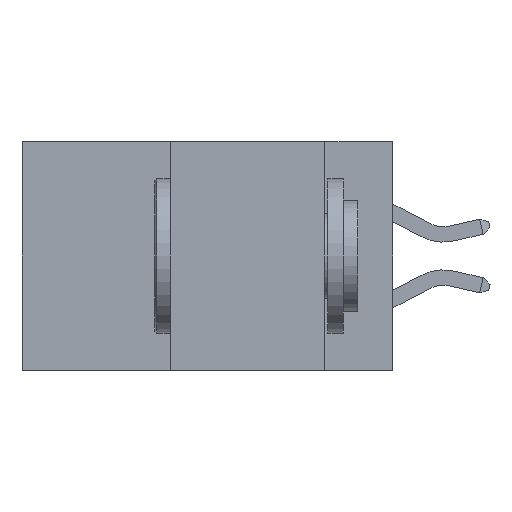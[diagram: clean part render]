
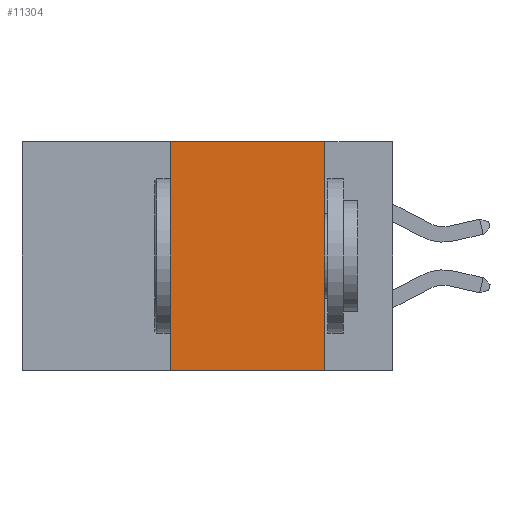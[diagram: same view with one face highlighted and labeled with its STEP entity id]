
A CAD part, left-side view. The second image highlights one B-rep face of the part: STEP entity #11304.
In plain terms, the highlighted planar face has unit normal (-1, 0, 0).
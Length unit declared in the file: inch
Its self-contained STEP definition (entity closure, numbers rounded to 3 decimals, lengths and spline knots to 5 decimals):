
#2167 = VECTOR ( 'NONE', #12149, 39.37008 ) ;
#3644 = EDGE_LOOP ( 'NONE', ( #26997, #8917, #14681, #18625 ) ) ;
#3926 = CARTESIAN_POINT ( 'NONE',  ( 0., 0.11, -0.37 ) ) ;
#5124 = EDGE_CURVE ( 'NONE', #15051, #18869, #25677, .T. ) ;
#5233 = CARTESIAN_POINT ( 'NONE',  ( 0., 0.6, 0. ) ) ;
#6805 = CARTESIAN_POINT ( 'NONE',  ( 0., 0.11, 0. ) ) ;
#6929 = EDGE_CURVE ( 'NONE', #10120, #15051, #9882, .T. ) ;
#7617 = LINE ( 'NONE', #21318, #2167 ) ;
#8111 = EDGE_CURVE ( 'NONE', #18869, #15556, #28634, .T. ) ;
#8841 = FACE_OUTER_BOUND ( 'NONE', #3644, .T. ) ;
#8917 = ORIENTED_EDGE ( 'NONE', *, *, #5124, .F. ) ;
#9882 = LINE ( 'NONE', #10503, #22283 ) ;
#10120 = VERTEX_POINT ( 'NONE', #28570 ) ;
#10503 = CARTESIAN_POINT ( 'NONE',  ( 0., 0.36, 0. ) ) ;
#10756 = CARTESIAN_POINT ( 'NONE',  ( 0., 0.6, 0. ) ) ;
#11304 = ADVANCED_FACE ( 'NONE', ( #8841 ), #28415, .F. ) ;
#11865 = DIRECTION ( 'NONE',  ( 1., 0., 0. ) ) ;
#12149 = DIRECTION ( 'NONE',  ( 0., -1., 0. ) ) ;
#13321 = EDGE_CURVE ( 'NONE', #10120, #15556, #7617, .T. ) ;
#14681 = ORIENTED_EDGE ( 'NONE', *, *, #6929, .F. ) ;
#15051 = VERTEX_POINT ( 'NONE', #24729 ) ;
#15556 = VERTEX_POINT ( 'NONE', #3926 ) ;
#16739 = DIRECTION ( 'NONE',  ( 0., 0., -1. ) ) ;
#17012 = VECTOR ( 'NONE', #26314, 39.37008 ) ;
#18625 = ORIENTED_EDGE ( 'NONE', *, *, #13321, .T. ) ;
#18869 = VERTEX_POINT ( 'NONE', #24136 ) ;
#21318 = CARTESIAN_POINT ( 'NONE',  ( 0., 0.6, -0.37 ) ) ;
#22283 = VECTOR ( 'NONE', #26687, 39.37008 ) ;
#24136 = CARTESIAN_POINT ( 'NONE',  ( 0., 0.11, 0. ) ) ;
#24729 = CARTESIAN_POINT ( 'NONE',  ( 0., 0.36, 0. ) ) ;
#24951 = VECTOR ( 'NONE', #27026, 39.37008 ) ;
#25677 = LINE ( 'NONE', #10756, #24951 ) ;
#26314 = DIRECTION ( 'NONE',  ( 0., 0., -1. ) ) ;
#26687 = DIRECTION ( 'NONE',  ( 0., 0., 1. ) ) ;
#26997 = ORIENTED_EDGE ( 'NONE', *, *, #8111, .F. ) ;
#27026 = DIRECTION ( 'NONE',  ( 0., -1., 0. ) ) ;
#28415 = PLANE ( 'NONE',  #28551 ) ;
#28551 = AXIS2_PLACEMENT_3D ( 'NONE', #5233, #11865, #16739 ) ;
#28570 = CARTESIAN_POINT ( 'NONE',  ( 0., 0.36, -0.37 ) ) ;
#28634 = LINE ( 'NONE', #6805, #17012 ) ;
